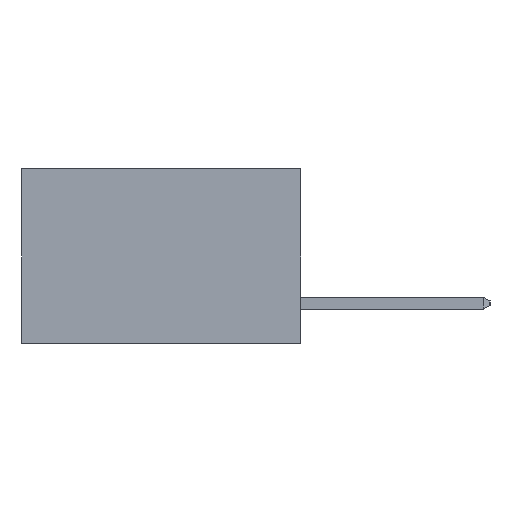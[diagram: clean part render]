
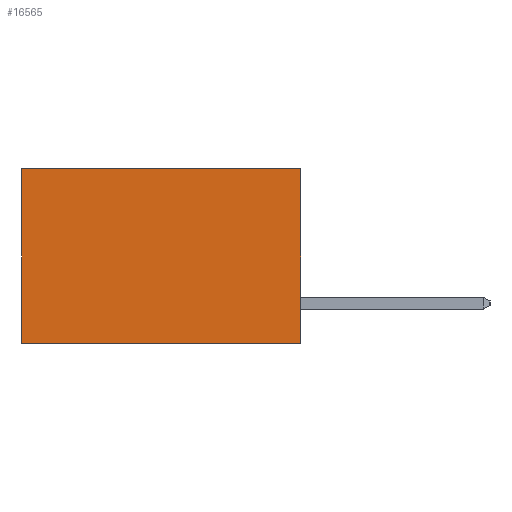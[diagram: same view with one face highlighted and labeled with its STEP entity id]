
A CAD part, left-side view. The second image highlights one B-rep face of the part: STEP entity #16565.
In plain terms, the highlighted planar face has unit normal (-1, 0, 0).
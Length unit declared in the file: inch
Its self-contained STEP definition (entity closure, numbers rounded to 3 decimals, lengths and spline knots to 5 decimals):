
#78 = LINE ( 'NONE', #6212, #21236 ) ;
#407 = VERTEX_POINT ( 'NONE', #503 ) ;
#503 = CARTESIAN_POINT ( 'NONE',  ( 0.277, 0., -0.37 ) ) ;
#906 = EDGE_CURVE ( 'NONE', #25533, #4882, #22213, .T. ) ;
#1342 = AXIS2_PLACEMENT_3D ( 'NONE', #19975, #21936, #9811 ) ;
#4882 = VERTEX_POINT ( 'NONE', #19333 ) ;
#5990 = VECTOR ( 'NONE', #21038, 39.37008 ) ;
#6075 = FACE_OUTER_BOUND ( 'NONE', #11519, .T. ) ;
#6212 = CARTESIAN_POINT ( 'NONE',  ( 0.277, 0., -0.37 ) ) ;
#6614 = CARTESIAN_POINT ( 'NONE',  ( 0.277, 0.59, -0.37 ) ) ;
#7234 = LINE ( 'NONE', #23575, #22766 ) ;
#9811 = DIRECTION ( 'NONE',  ( 0., 0., -1. ) ) ;
#10845 = VERTEX_POINT ( 'NONE', #6614 ) ;
#11389 = ORIENTED_EDGE ( 'NONE', *, *, #22843, .T. ) ;
#11519 = EDGE_LOOP ( 'NONE', ( #11389, #17810, #12368, #12055 ) ) ;
#12055 = ORIENTED_EDGE ( 'NONE', *, *, #906, .T. ) ;
#12368 = ORIENTED_EDGE ( 'NONE', *, *, #23123, .F. ) ;
#12567 = EDGE_CURVE ( 'NONE', #407, #10845, #21244, .T. ) ;
#13587 = DIRECTION ( 'NONE',  ( 0., 0., -1. ) ) ;
#15036 = CARTESIAN_POINT ( 'NONE',  ( 0.277, 0., 0. ) ) ;
#16309 = CARTESIAN_POINT ( 'NONE',  ( 0.277, 0., -0.37 ) ) ;
#16565 = ADVANCED_FACE ( 'NONE', ( #6075 ), #17960, .F. ) ;
#16890 = DIRECTION ( 'NONE',  ( 0., 0., -1. ) ) ;
#17810 = ORIENTED_EDGE ( 'NONE', *, *, #12567, .F. ) ;
#17960 = PLANE ( 'NONE',  #1342 ) ;
#19333 = CARTESIAN_POINT ( 'NONE',  ( 0.277, 0.59, 0. ) ) ;
#19975 = CARTESIAN_POINT ( 'NONE',  ( 0.277, 0., -0.37 ) ) ;
#20460 = DIRECTION ( 'NONE',  ( 0., 1., 0. ) ) ;
#20781 = CARTESIAN_POINT ( 'NONE',  ( 0.277, 0., 0. ) ) ;
#21038 = DIRECTION ( 'NONE',  ( 0., 1., 0. ) ) ;
#21236 = VECTOR ( 'NONE', #16890, 39.37008 ) ;
#21244 = LINE ( 'NONE', #16309, #25170 ) ;
#21936 = DIRECTION ( 'NONE',  ( 1., 0., 0. ) ) ;
#22213 = LINE ( 'NONE', #20781, #5990 ) ;
#22766 = VECTOR ( 'NONE', #13587, 39.37008 ) ;
#22843 = EDGE_CURVE ( 'NONE', #4882, #10845, #7234, .T. ) ;
#23123 = EDGE_CURVE ( 'NONE', #25533, #407, #78, .T. ) ;
#23575 = CARTESIAN_POINT ( 'NONE',  ( 0.277, 0.59, -0.37 ) ) ;
#25170 = VECTOR ( 'NONE', #20460, 39.37008 ) ;
#25533 = VERTEX_POINT ( 'NONE', #15036 ) ;
